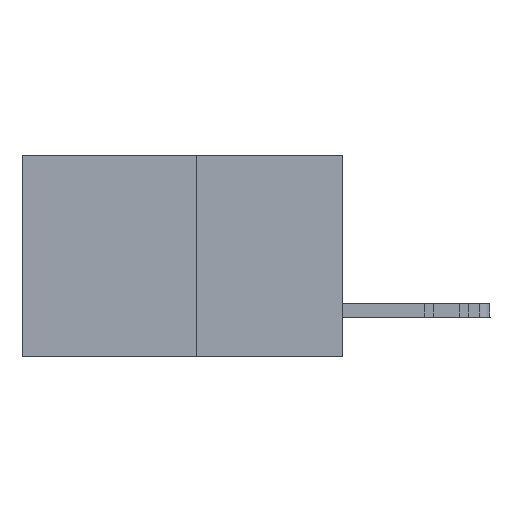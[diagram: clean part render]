
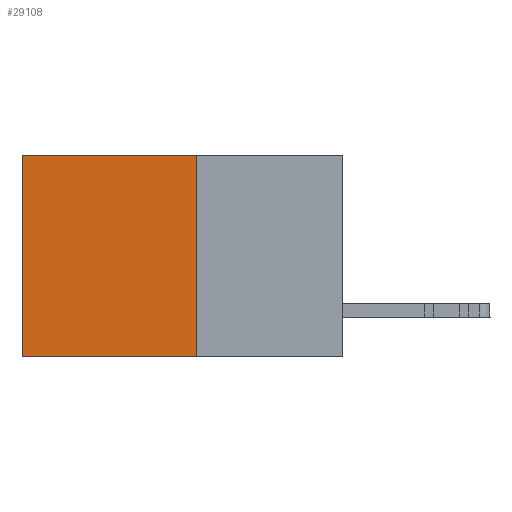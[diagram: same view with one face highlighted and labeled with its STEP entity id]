
A CAD part, left-side view. The second image highlights one B-rep face of the part: STEP entity #29108.
In plain terms, the highlighted planar face has unit normal (-1, 0, 0).
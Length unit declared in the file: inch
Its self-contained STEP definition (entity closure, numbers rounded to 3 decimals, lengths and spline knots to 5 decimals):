
#407 = CARTESIAN_POINT ( 'NONE',  ( 0.277, 0.27, -0.37 ) ) ;
#627 = VERTEX_POINT ( 'NONE', #13260 ) ;
#2039 = LINE ( 'NONE', #9564, #10960 ) ;
#2065 = VERTEX_POINT ( 'NONE', #407 ) ;
#5146 = CARTESIAN_POINT ( 'NONE',  ( 0.277, 0.59, 0. ) ) ;
#5589 = DIRECTION ( 'NONE',  ( 0., 0., -1. ) ) ;
#5966 = EDGE_CURVE ( 'NONE', #11861, #19747, #31536, .T. ) ;
#6058 = CARTESIAN_POINT ( 'NONE',  ( 0.277, 0.27, -0.37 ) ) ;
#7155 = EDGE_CURVE ( 'NONE', #627, #2065, #26793, .T. ) ;
#7748 = CARTESIAN_POINT ( 'NONE',  ( 0.277, 0.59, -0.37 ) ) ;
#9298 = ORIENTED_EDGE ( 'NONE', *, *, #7155, .F. ) ;
#9402 = DIRECTION ( 'NONE',  ( 0., 1., 0. ) ) ;
#9564 = CARTESIAN_POINT ( 'NONE',  ( 0.277, 0.27, 0. ) ) ;
#10960 = VECTOR ( 'NONE', #9402, 39.37008 ) ;
#11150 = VECTOR ( 'NONE', #5589, 39.37008 ) ;
#11861 = VERTEX_POINT ( 'NONE', #5146 ) ;
#12773 = DIRECTION ( 'NONE',  ( 0., 0., -1. ) ) ;
#12792 = EDGE_CURVE ( 'NONE', #2065, #19747, #19607, .T. ) ;
#13260 = CARTESIAN_POINT ( 'NONE',  ( 0.277, 0.27, 0. ) ) ;
#15378 = VECTOR ( 'NONE', #12773, 39.37008 ) ;
#16186 = CARTESIAN_POINT ( 'NONE',  ( 0.277, 0.27, -0.37 ) ) ;
#16667 = DIRECTION ( 'NONE',  ( 1., 0., 0. ) ) ;
#17337 = CARTESIAN_POINT ( 'NONE',  ( 0.277, 0.27, -0.37 ) ) ;
#18013 = EDGE_CURVE ( 'NONE', #627, #11861, #2039, .T. ) ;
#18216 = AXIS2_PLACEMENT_3D ( 'NONE', #6058, #16667, #27262 ) ;
#19272 = PLANE ( 'NONE',  #18216 ) ;
#19607 = LINE ( 'NONE', #17337, #30894 ) ;
#19747 = VERTEX_POINT ( 'NONE', #24545 ) ;
#21421 = ORIENTED_EDGE ( 'NONE', *, *, #18013, .T. ) ;
#24485 = EDGE_LOOP ( 'NONE', ( #30444, #33787, #9298, #21421 ) ) ;
#24545 = CARTESIAN_POINT ( 'NONE',  ( 0.277, 0.59, -0.37 ) ) ;
#26793 = LINE ( 'NONE', #16186, #11150 ) ;
#27262 = DIRECTION ( 'NONE',  ( 0., 0., -1. ) ) ;
#27264 = DIRECTION ( 'NONE',  ( 0., 1., 0. ) ) ;
#27589 = FACE_OUTER_BOUND ( 'NONE', #24485, .T. ) ;
#29108 = ADVANCED_FACE ( 'NONE', ( #27589 ), #19272, .F. ) ;
#30444 = ORIENTED_EDGE ( 'NONE', *, *, #5966, .T. ) ;
#30894 = VECTOR ( 'NONE', #27264, 39.37008 ) ;
#31536 = LINE ( 'NONE', #7748, #15378 ) ;
#33787 = ORIENTED_EDGE ( 'NONE', *, *, #12792, .F. ) ;
